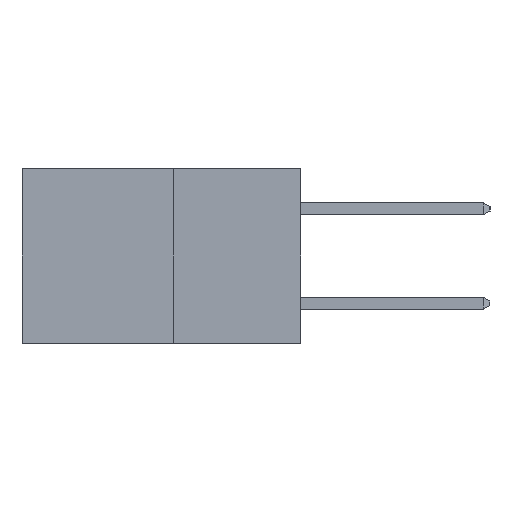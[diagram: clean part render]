
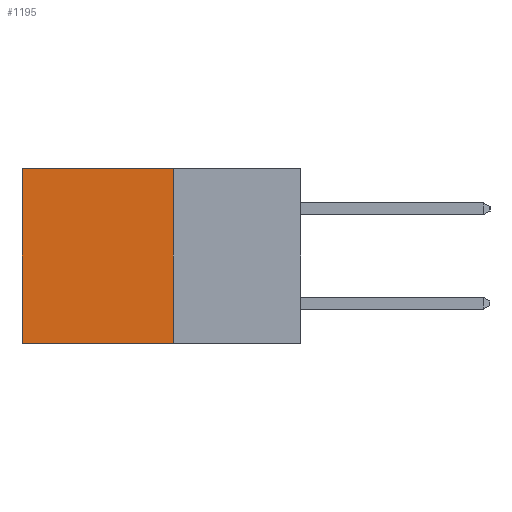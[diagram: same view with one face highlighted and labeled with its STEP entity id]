
A CAD part, left-side view. The second image highlights one B-rep face of the part: STEP entity #1195.
In plain terms, the highlighted planar face has unit normal (-1, 0, 0).
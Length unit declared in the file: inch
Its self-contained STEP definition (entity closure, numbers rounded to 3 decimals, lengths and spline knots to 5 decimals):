
#259 = DIRECTION ( 'NONE',  ( 0., 1., 0. ) ) ;
#319 = VERTEX_POINT ( 'NONE', #12625 ) ;
#1195 = ADVANCED_FACE ( 'NONE', ( #16628 ), #9537, .F. ) ;
#1918 = ORIENTED_EDGE ( 'NONE', *, *, #15758, .F. ) ;
#2150 = EDGE_CURVE ( 'NONE', #3237, #319, #17046, .T. ) ;
#2337 = VECTOR ( 'NONE', #4998, 39.37008 ) ;
#3237 = VERTEX_POINT ( 'NONE', #17091 ) ;
#3587 = CARTESIAN_POINT ( 'NONE',  ( 0.277, 0.59, 0. ) ) ;
#3939 = ORIENTED_EDGE ( 'NONE', *, *, #6482, .T. ) ;
#4001 = CARTESIAN_POINT ( 'NONE',  ( 0.277, 0.27, -0.37 ) ) ;
#4710 = CARTESIAN_POINT ( 'NONE',  ( 0.277, 0.27, 0. ) ) ;
#4846 = LINE ( 'NONE', #16824, #15940 ) ;
#4998 = DIRECTION ( 'NONE',  ( 0., 0., -1. ) ) ;
#6307 = VERTEX_POINT ( 'NONE', #15019 ) ;
#6482 = EDGE_CURVE ( 'NONE', #7671, #319, #4846, .T. ) ;
#6707 = VECTOR ( 'NONE', #259, 39.37008 ) ;
#6856 = EDGE_LOOP ( 'NONE', ( #3939, #14914, #1918, #18786 ) ) ;
#7059 = AXIS2_PLACEMENT_3D ( 'NONE', #4001, #12718, #15253 ) ;
#7671 = VERTEX_POINT ( 'NONE', #3587 ) ;
#9537 = PLANE ( 'NONE',  #7059 ) ;
#9968 = CARTESIAN_POINT ( 'NONE',  ( 0.277, 0.27, -0.37 ) ) ;
#10885 = DIRECTION ( 'NONE',  ( 0., 1., 0. ) ) ;
#12625 = CARTESIAN_POINT ( 'NONE',  ( 0.277, 0.59, -0.37 ) ) ;
#12645 = VECTOR ( 'NONE', #10885, 39.37008 ) ;
#12718 = DIRECTION ( 'NONE',  ( 1., 0., 0. ) ) ;
#13628 = CARTESIAN_POINT ( 'NONE',  ( 0.277, 0.27, -0.37 ) ) ;
#13883 = LINE ( 'NONE', #13628, #2337 ) ;
#14353 = EDGE_CURVE ( 'NONE', #6307, #7671, #14380, .T. ) ;
#14380 = LINE ( 'NONE', #4710, #6707 ) ;
#14914 = ORIENTED_EDGE ( 'NONE', *, *, #2150, .F. ) ;
#15019 = CARTESIAN_POINT ( 'NONE',  ( 0.277, 0.27, 0. ) ) ;
#15253 = DIRECTION ( 'NONE',  ( 0., 0., -1. ) ) ;
#15758 = EDGE_CURVE ( 'NONE', #6307, #3237, #13883, .T. ) ;
#15940 = VECTOR ( 'NONE', #18374, 39.37008 ) ;
#16628 = FACE_OUTER_BOUND ( 'NONE', #6856, .T. ) ;
#16824 = CARTESIAN_POINT ( 'NONE',  ( 0.277, 0.59, -0.37 ) ) ;
#17046 = LINE ( 'NONE', #9968, #12645 ) ;
#17091 = CARTESIAN_POINT ( 'NONE',  ( 0.277, 0.27, -0.37 ) ) ;
#18374 = DIRECTION ( 'NONE',  ( 0., 0., -1. ) ) ;
#18786 = ORIENTED_EDGE ( 'NONE', *, *, #14353, .T. ) ;
